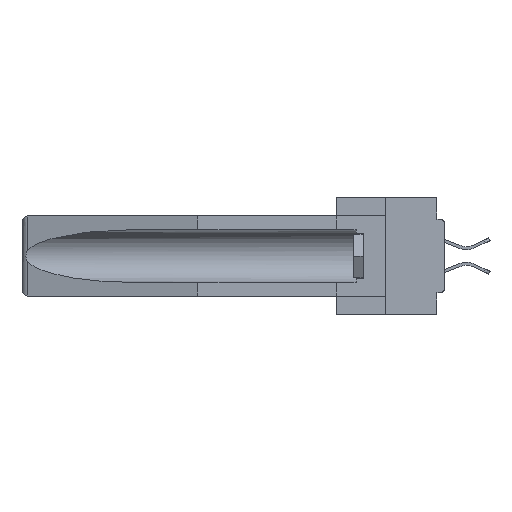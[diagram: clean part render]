
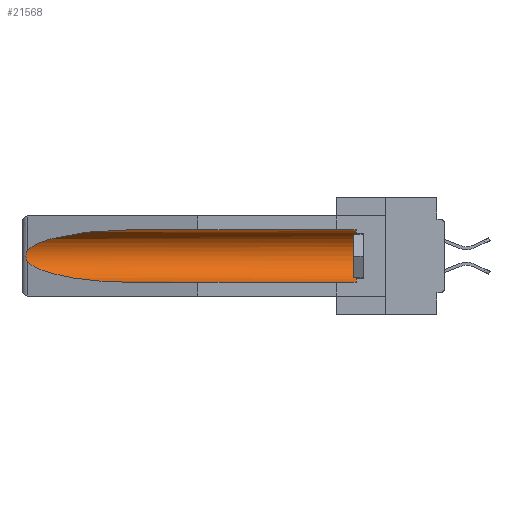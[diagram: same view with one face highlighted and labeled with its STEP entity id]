
A CAD part, left-side view. The second image highlights one B-rep face of the part: STEP entity #21568.
In plain terms, the highlighted cylindrical face has radius 2.857 mm (diameter 5.715 mm), a partial arc.
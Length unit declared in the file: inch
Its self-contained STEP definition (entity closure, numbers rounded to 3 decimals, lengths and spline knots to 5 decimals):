
#527 = CARTESIAN_POINT ( 'NONE',  ( 0.26537, 1.52718, -0.14972 ) ) ;
#1274 = EDGE_CURVE ( 'NONE', #20601, #37569, #30876, .T. ) ;
#2565 = DIRECTION ( 'NONE',  ( 0., 0., 1. ) ) ;
#3519 = VERTEX_POINT ( 'NONE', #527 ) ;
#4966 = CARTESIAN_POINT ( 'NONE',  ( 0.155, -0.30754, -0.1715 ) ) ;
#5157 = CARTESIAN_POINT ( 'NONE',  ( 0.155, 1.07973, -0.059 ) ) ;
#5294 = CARTESIAN_POINT ( 'NONE',  ( 0.21114, 1.30732, -0.059 ) ) ;
#6100 = ORIENTED_EDGE ( 'NONE', *, *, #38579, .T. ) ;
#7888 = DIRECTION ( 'NONE',  ( 0., 1., 0. ) ) ;
#8036 = CARTESIAN_POINT ( 'NONE',  ( 0.155, 0.126, -0.059 ) ) ;
#8459 = CARTESIAN_POINT ( 'NONE',  ( 0.26537, 1.52718, -0.14972 ) ) ;
#9959 = ORIENTED_EDGE ( 'NONE', *, *, #1274, .T. ) ;
#10413 = CARTESIAN_POINT ( 'NONE',  ( 0.2673, 1.53269, -0.17917 ) ) ;
#10538 = CARTESIAN_POINT ( 'NONE',  ( 0.2675, 1.53308, -0.17534 ) ) ;
#10801 = DIRECTION ( 'NONE',  ( 0., 1., 0. ) ) ;
#11236 = CARTESIAN_POINT ( 'NONE',  ( 0.25451, 1.48313, -0.09465 ) ) ;
#12109 = VERTEX_POINT ( 'NONE', #22807 ) ;
#14716 = ORIENTED_EDGE ( 'NONE', *, *, #16104, .T. ) ;
#15941 = EDGE_CURVE ( 'NONE', #12109, #37569, #22784, .T. ) ;
#16104 = EDGE_CURVE ( 'NONE', #21045, #3519, #24958, .T. ) ;
#16603 = CARTESIAN_POINT ( 'NONE',  ( 0.2673, 1.5327, -0.16383 ) ) ;
#16976 = CARTESIAN_POINT ( 'NONE',  ( 0.26537, 1.52718, -0.19328 ) ) ;
#17063 = ORIENTED_EDGE ( 'NONE', *, *, #19696, .T. ) ;
#17742 = CIRCLE ( 'NONE', #19613, 0.1125 ) ;
#19613 = AXIS2_PLACEMENT_3D ( 'NONE', #20749, #33102, #2565 ) ;
#19696 = EDGE_CURVE ( 'NONE', #12109, #34642, #17742, .T. ) ;
#20601 = VERTEX_POINT ( 'NONE', #20630 ) ;
#20630 = CARTESIAN_POINT ( 'NONE',  ( 0.26537, 1.52718, -0.19328 ) ) ;
#20749 = CARTESIAN_POINT ( 'NONE',  ( 0.155, 0.126, -0.1715 ) ) ;
#21045 = VERTEX_POINT ( 'NONE', #35090 ) ;
#21568 = ADVANCED_FACE ( 'NONE', ( #37223 ), #29097, .F. ) ;
#22369 = CARTESIAN_POINT ( 'NONE',  ( 0.155, -0.30754, -0.284 ) ) ;
#22614 = CARTESIAN_POINT ( 'NONE',  ( 0.26597, 1.5296, -0.19026 ) ) ;
#22709 = AXIS2_PLACEMENT_3D ( 'NONE', #4966, #7888, #29223 ) ;
#22784 = LINE ( 'NONE', #22369, #35265 ) ;
#22807 = CARTESIAN_POINT ( 'NONE',  ( 0.155, 0.126, -0.284 ) ) ;
#23011 = CARTESIAN_POINT ( 'NONE',  ( 0.2675, 1.53308, -0.16763 ) ) ;
#23118 = CARTESIAN_POINT ( 'NONE',  ( 0.155, 1.07973, -0.284 ) ) ;
#24506 = CARTESIAN_POINT ( 'NONE',  ( 0.155, 1.07973, -0.284 ) ) ;
#24958 =( BOUNDED_CURVE ( )  B_SPLINE_CURVE ( 3, ( #5157, #5294, #11236, #8459 ),
 .UNSPECIFIED., .F., .T. ) 
 B_SPLINE_CURVE_WITH_KNOTS ( ( 4, 4 ),
 ( 4.71239, 6.08839 ),
 .UNSPECIFIED. ) 
 CURVE ( )  GEOMETRIC_REPRESENTATION_ITEM ( )  RATIONAL_B_SPLINE_CURVE ( ( 1., 0.848, 0.848, 1. ) ) 
 REPRESENTATION_ITEM ( '' )  );
#25357 = LINE ( 'NONE', #27480, #36373 ) ;
#25710 = CARTESIAN_POINT ( 'NONE',  ( 0.26537, 1.52718, -0.19328 ) ) ;
#26472 = CARTESIAN_POINT ( 'NONE',  ( 0.21114, 1.30732, -0.284 ) ) ;
#27480 = CARTESIAN_POINT ( 'NONE',  ( 0.155, -0.30754, -0.059 ) ) ;
#28416 = ORIENTED_EDGE ( 'NONE', *, *, #15941, .F. ) ;
#29097 = CYLINDRICAL_SURFACE ( 'NONE', #22709, 0.1125 ) ;
#29223 = DIRECTION ( 'NONE',  ( 0., 0., 1. ) ) ;
#29445 = CARTESIAN_POINT ( 'NONE',  ( 0.25451, 1.48313, -0.24835 ) ) ;
#30702 = DIRECTION ( 'NONE',  ( 0., 1., 0. ) ) ;
#30876 =( BOUNDED_CURVE ( )  B_SPLINE_CURVE ( 3, ( #16976, #29445, #26472, #23118 ),
 .UNSPECIFIED., .F., .F. ) 
 B_SPLINE_CURVE_WITH_KNOTS ( ( 4, 4 ),
 ( 0.1948, 1.5708 ),
 .UNSPECIFIED. ) 
 CURVE ( )  GEOMETRIC_REPRESENTATION_ITEM ( )  RATIONAL_B_SPLINE_CURVE ( ( 1., 0.848, 0.848, 1. ) ) 
 REPRESENTATION_ITEM ( '' )  );
#31639 = CARTESIAN_POINT ( 'NONE',  ( 0.26654, 1.53092, -0.15636 ) ) ;
#31902 = CARTESIAN_POINT ( 'NONE',  ( 0.26655, 1.53094, -0.18657 ) ) ;
#32950 = ORIENTED_EDGE ( 'NONE', *, *, #35998, .T. ) ;
#33102 = DIRECTION ( 'NONE',  ( 0., -1., 0. ) ) ;
#34642 = VERTEX_POINT ( 'NONE', #8036 ) ;
#34969 = CARTESIAN_POINT ( 'NONE',  ( 0.26597, 1.52961, -0.15275 ) ) ;
#35090 = CARTESIAN_POINT ( 'NONE',  ( 0.155, 1.07973, -0.059 ) ) ;
#35265 = VECTOR ( 'NONE', #10801, 39.37008 ) ;
#35998 = EDGE_CURVE ( 'NONE', #34642, #21045, #25357, .T. ) ;
#36196 = EDGE_LOOP ( 'NONE', ( #14716, #6100, #9959, #28416, #17063, #32950 ) ) ;
#36373 = VECTOR ( 'NONE', #30702, 39.37008 ) ;
#37223 = FACE_OUTER_BOUND ( 'NONE', #36196, .T. ) ;
#37569 = VERTEX_POINT ( 'NONE', #24506 ) ;
#38301 = CARTESIAN_POINT ( 'NONE',  ( 0.26537, 1.52718, -0.14972 ) ) ;
#38579 = EDGE_CURVE ( 'NONE', #3519, #20601, #39174, .T. ) ;
#39174 = B_SPLINE_CURVE_WITH_KNOTS ( 'NONE', 3,
 ( #38301, #34969, #31639, #16603, #23011, #10538, #10413, #31902, #22614, #25710 ),
 .UNSPECIFIED., .F., .F.,
 ( 4, 2, 2, 2, 4 ),
 ( 0., 0.00029, 0.00058, 0.00087, 0.00117 ),
 .UNSPECIFIED. ) ;
